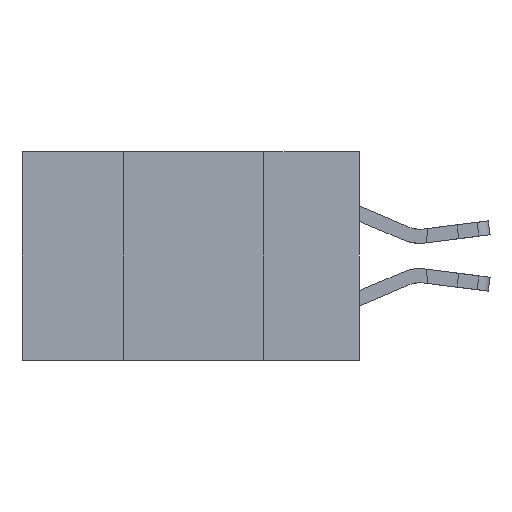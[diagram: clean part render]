
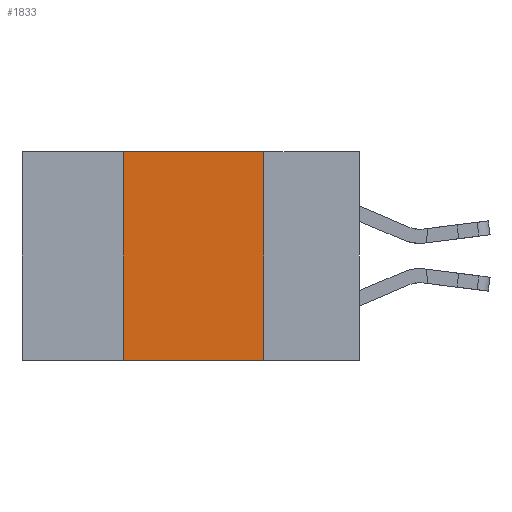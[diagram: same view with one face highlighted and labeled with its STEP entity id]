
A CAD part, left-side view. The second image highlights one B-rep face of the part: STEP entity #1833.
In plain terms, the highlighted planar face has unit normal (-1, 0, 0).
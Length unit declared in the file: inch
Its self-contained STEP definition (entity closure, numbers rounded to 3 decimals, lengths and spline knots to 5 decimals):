
#641 = DIRECTION ( 'NONE',  ( 0., 0., -1. ) ) ;
#1649 = ORIENTED_EDGE ( 'NONE', *, *, #10086, .F. ) ;
#1833 = ADVANCED_FACE ( 'NONE', ( #3587 ), #29557, .F. ) ;
#2940 = VECTOR ( 'NONE', #32877, 39.37008 ) ;
#3151 = LINE ( 'NONE', #4603, #30323 ) ;
#3587 = FACE_OUTER_BOUND ( 'NONE', #33028, .T. ) ;
#4070 = VECTOR ( 'NONE', #22529, 39.37008 ) ;
#4479 = DIRECTION ( 'NONE',  ( 0., -1., 0. ) ) ;
#4603 = CARTESIAN_POINT ( 'NONE',  ( 0., 0.6, -0.37 ) ) ;
#5293 = CARTESIAN_POINT ( 'NONE',  ( 0., 0.42, -0.37 ) ) ;
#6279 = CARTESIAN_POINT ( 'NONE',  ( 0., 0.17, 0. ) ) ;
#8708 = VERTEX_POINT ( 'NONE', #29815 ) ;
#8766 = DIRECTION ( 'NONE',  ( 0., 0., -1. ) ) ;
#9182 = ORIENTED_EDGE ( 'NONE', *, *, #19505, .F. ) ;
#10086 = EDGE_CURVE ( 'NONE', #23517, #29793, #31977, .T. ) ;
#13568 = AXIS2_PLACEMENT_3D ( 'NONE', #13806, #16464, #641 ) ;
#13806 = CARTESIAN_POINT ( 'NONE',  ( 0., 0.6, 0. ) ) ;
#14597 = CARTESIAN_POINT ( 'NONE',  ( 0., 0.42, 0. ) ) ;
#16152 = ORIENTED_EDGE ( 'NONE', *, *, #26773, .F. ) ;
#16464 = DIRECTION ( 'NONE',  ( 1., 0., 0. ) ) ;
#18794 = ORIENTED_EDGE ( 'NONE', *, *, #21630, .T. ) ;
#19505 = EDGE_CURVE ( 'NONE', #29793, #8708, #19847, .T. ) ;
#19847 = LINE ( 'NONE', #24588, #33657 ) ;
#21042 = CARTESIAN_POINT ( 'NONE',  ( 0., 0.42, 0. ) ) ;
#21630 = EDGE_CURVE ( 'NONE', #28877, #8708, #3151, .T. ) ;
#22353 = LINE ( 'NONE', #14597, #2940 ) ;
#22529 = DIRECTION ( 'NONE',  ( 0., -1., 0. ) ) ;
#23517 = VERTEX_POINT ( 'NONE', #21042 ) ;
#24588 = CARTESIAN_POINT ( 'NONE',  ( 0., 0.17, 0. ) ) ;
#26773 = EDGE_CURVE ( 'NONE', #28877, #23517, #22353, .T. ) ;
#28877 = VERTEX_POINT ( 'NONE', #5293 ) ;
#29557 = PLANE ( 'NONE',  #13568 ) ;
#29793 = VERTEX_POINT ( 'NONE', #6279 ) ;
#29815 = CARTESIAN_POINT ( 'NONE',  ( 0., 0.17, -0.37 ) ) ;
#30323 = VECTOR ( 'NONE', #4479, 39.37008 ) ;
#31977 = LINE ( 'NONE', #32845, #4070 ) ;
#32845 = CARTESIAN_POINT ( 'NONE',  ( 0., 0.6, 0. ) ) ;
#32877 = DIRECTION ( 'NONE',  ( 0., 0., 1. ) ) ;
#33028 = EDGE_LOOP ( 'NONE', ( #9182, #1649, #16152, #18794 ) ) ;
#33657 = VECTOR ( 'NONE', #8766, 39.37008 ) ;
